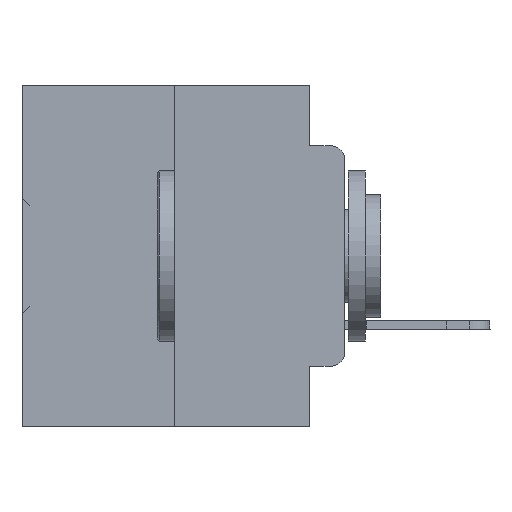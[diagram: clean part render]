
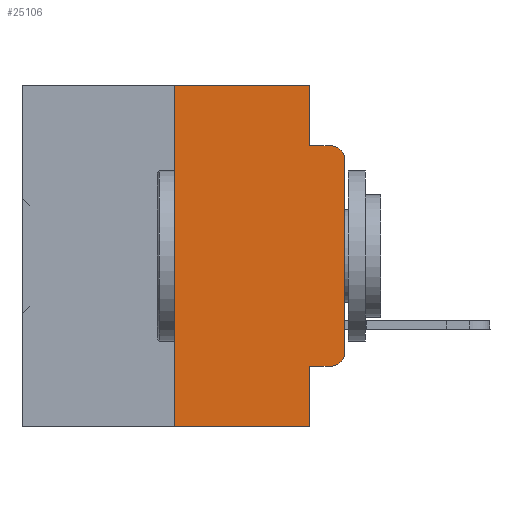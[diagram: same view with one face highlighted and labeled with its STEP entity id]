
A CAD part, left-side view. The second image highlights one B-rep face of the part: STEP entity #25106.
In plain terms, the highlighted planar face has unit normal (-1, 0, 0).
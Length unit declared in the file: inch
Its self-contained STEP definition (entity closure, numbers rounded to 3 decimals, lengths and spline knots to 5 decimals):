
#1083 = EDGE_CURVE ( 'NONE', #20286, #31604, #16073, .T. ) ;
#1217 = AXIS2_PLACEMENT_3D ( 'NONE', #29743, #11749, #23890 ) ;
#1249 = ORIENTED_EDGE ( 'NONE', *, *, #6291, .T. ) ;
#1398 = CARTESIAN_POINT ( 'NONE',  ( 0., 0.02, -0.0885 ) ) ;
#1804 = CARTESIAN_POINT ( 'NONE',  ( 0., 0.25, 0. ) ) ;
#2836 = VERTEX_POINT ( 'NONE', #11059 ) ;
#2842 = ORIENTED_EDGE ( 'NONE', *, *, #24667, .T. ) ;
#4216 = ORIENTED_EDGE ( 'NONE', *, *, #34465, .T. ) ;
#4657 = EDGE_CURVE ( 'NONE', #28585, #14740, #22027, .T. ) ;
#5127 = DIRECTION ( 'NONE',  ( 1., 0., 0. ) ) ;
#5348 = LINE ( 'NONE', #27238, #24746 ) ;
#6280 = LINE ( 'NONE', #24046, #9127 ) ;
#6291 = EDGE_CURVE ( 'NONE', #21376, #9202, #21209, .T. ) ;
#8131 = EDGE_CURVE ( 'NONE', #38705, #28585, #34375, .T. ) ;
#8152 = CIRCLE ( 'NONE', #1217, 0.02 ) ;
#8681 = CARTESIAN_POINT ( 'NONE',  ( 0., 0.473, 0. ) ) ;
#9045 = CARTESIAN_POINT ( 'NONE',  ( 0., 0., 0. ) ) ;
#9127 = VECTOR ( 'NONE', #21553, 39.37008 ) ;
#9202 = VERTEX_POINT ( 'NONE', #13160 ) ;
#10033 = CARTESIAN_POINT ( 'NONE',  ( 0., 0.25, -0.5 ) ) ;
#10964 = ORIENTED_EDGE ( 'NONE', *, *, #37237, .F. ) ;
#11059 = CARTESIAN_POINT ( 'NONE',  ( 0., 0., -0.1085 ) ) ;
#11312 = DIRECTION ( 'NONE',  ( 0., -1., 0. ) ) ;
#11742 = DIRECTION ( 'NONE',  ( 0., 0., -1. ) ) ;
#11749 = DIRECTION ( 'NONE',  ( -1., 0., 0. ) ) ;
#12705 = DIRECTION ( 'NONE',  ( -1., 0., 0. ) ) ;
#13160 = CARTESIAN_POINT ( 'NONE',  ( 0., 0.02, -0.4115 ) ) ;
#14740 = VERTEX_POINT ( 'NONE', #36125 ) ;
#15265 = EDGE_CURVE ( 'NONE', #20286, #38705, #21806, .T. ) ;
#15900 = CARTESIAN_POINT ( 'NONE',  ( 0., 0.051, -0.4115 ) ) ;
#16073 = LINE ( 'NONE', #26388, #38842 ) ;
#17696 = VERTEX_POINT ( 'NONE', #26432 ) ;
#18770 = CARTESIAN_POINT ( 'NONE',  ( 0., 0.051, 0. ) ) ;
#18968 = LINE ( 'NONE', #9045, #25130 ) ;
#20015 = ORIENTED_EDGE ( 'NONE', *, *, #15265, .F. ) ;
#20286 = VERTEX_POINT ( 'NONE', #10033 ) ;
#20347 = DIRECTION ( 'NONE',  ( 0., -1., 0. ) ) ;
#20524 = DIRECTION ( 'NONE',  ( 0., 0., 1. ) ) ;
#20731 = PLANE ( 'NONE',  #37053 ) ;
#20973 = CIRCLE ( 'NONE', #35784, 0.02 ) ;
#21209 = LINE ( 'NONE', #15900, #36855 ) ;
#21376 = VERTEX_POINT ( 'NONE', #35981 ) ;
#21553 = DIRECTION ( 'NONE',  ( 0., 0., -1. ) ) ;
#21806 = LINE ( 'NONE', #1804, #26053 ) ;
#22027 = LINE ( 'NONE', #36643, #38636 ) ;
#23890 = DIRECTION ( 'NONE',  ( 0., 0., -1. ) ) ;
#24046 = CARTESIAN_POINT ( 'NONE',  ( 0., 0.051, 0. ) ) ;
#24667 = EDGE_CURVE ( 'NONE', #9202, #17696, #20973, .T. ) ;
#24746 = VECTOR ( 'NONE', #30285, 39.37008 ) ;
#24853 = EDGE_LOOP ( 'NONE', ( #25397, #4216, #10964, #39164, #27827, #20015, #32656, #38286, #1249, #2842 ) ) ;
#25106 = ADVANCED_FACE ( 'NONE', ( #27071 ), #20731, .F. ) ;
#25130 = VECTOR ( 'NONE', #33274, 39.37008 ) ;
#25397 = ORIENTED_EDGE ( 'NONE', *, *, #35061, .T. ) ;
#26053 = VECTOR ( 'NONE', #20524, 39.37008 ) ;
#26388 = CARTESIAN_POINT ( 'NONE',  ( 0., 0.473, -0.5 ) ) ;
#26432 = CARTESIAN_POINT ( 'NONE',  ( 0., 0., -0.3915 ) ) ;
#27071 = FACE_OUTER_BOUND ( 'NONE', #24853, .T. ) ;
#27238 = CARTESIAN_POINT ( 'NONE',  ( 0., 0.051, -0.0885 ) ) ;
#27827 = ORIENTED_EDGE ( 'NONE', *, *, #8131, .F. ) ;
#28585 = VERTEX_POINT ( 'NONE', #18770 ) ;
#28720 = VECTOR ( 'NONE', #20347, 39.37008 ) ;
#29743 = CARTESIAN_POINT ( 'NONE',  ( 0., 0.02, -0.1085 ) ) ;
#29968 = CARTESIAN_POINT ( 'NONE',  ( 0., 0.25, 0. ) ) ;
#30285 = DIRECTION ( 'NONE',  ( 0., -1., 0. ) ) ;
#30682 = DIRECTION ( 'NONE',  ( 0., 0., -1. ) ) ;
#30812 = CARTESIAN_POINT ( 'NONE',  ( 0., 0.02, -0.3915 ) ) ;
#31604 = VERTEX_POINT ( 'NONE', #36095 ) ;
#31969 = CARTESIAN_POINT ( 'NONE',  ( 0., 0.473, 0. ) ) ;
#32656 = ORIENTED_EDGE ( 'NONE', *, *, #1083, .T. ) ;
#33274 = DIRECTION ( 'NONE',  ( 0., 0., 1. ) ) ;
#33872 = DIRECTION ( 'NONE',  ( 0., 0., -1. ) ) ;
#34375 = LINE ( 'NONE', #31969, #28720 ) ;
#34465 = EDGE_CURVE ( 'NONE', #2836, #36945, #8152, .T. ) ;
#35061 = EDGE_CURVE ( 'NONE', #17696, #2836, #18968, .T. ) ;
#35624 = DIRECTION ( 'NONE',  ( 0., -1., 0. ) ) ;
#35784 = AXIS2_PLACEMENT_3D ( 'NONE', #30812, #12705, #33872 ) ;
#35981 = CARTESIAN_POINT ( 'NONE',  ( 0., 0.051, -0.4115 ) ) ;
#36095 = CARTESIAN_POINT ( 'NONE',  ( 0., 0.051, -0.5 ) ) ;
#36125 = CARTESIAN_POINT ( 'NONE',  ( 0., 0.051, -0.0885 ) ) ;
#36643 = CARTESIAN_POINT ( 'NONE',  ( 0., 0.051, 0. ) ) ;
#36855 = VECTOR ( 'NONE', #35624, 39.37008 ) ;
#36945 = VERTEX_POINT ( 'NONE', #1398 ) ;
#37053 = AXIS2_PLACEMENT_3D ( 'NONE', #8681, #5127, #11742 ) ;
#37237 = EDGE_CURVE ( 'NONE', #14740, #36945, #5348, .T. ) ;
#37299 = EDGE_CURVE ( 'NONE', #21376, #31604, #6280, .T. ) ;
#38286 = ORIENTED_EDGE ( 'NONE', *, *, #37299, .F. ) ;
#38636 = VECTOR ( 'NONE', #30682, 39.37008 ) ;
#38705 = VERTEX_POINT ( 'NONE', #29968 ) ;
#38842 = VECTOR ( 'NONE', #11312, 39.37008 ) ;
#39164 = ORIENTED_EDGE ( 'NONE', *, *, #4657, .F. ) ;
